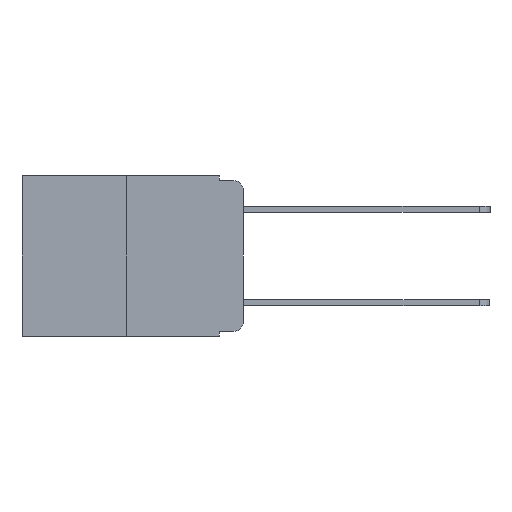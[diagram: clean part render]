
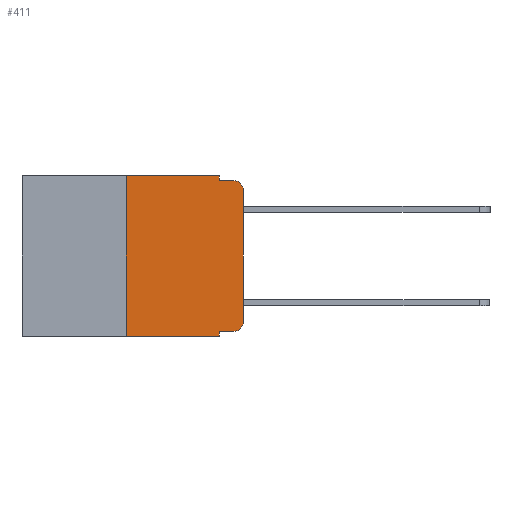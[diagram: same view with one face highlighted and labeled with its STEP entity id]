
A CAD part, left-side view. The second image highlights one B-rep face of the part: STEP entity #411.
In plain terms, the highlighted planar face has unit normal (-1, 0, 0).
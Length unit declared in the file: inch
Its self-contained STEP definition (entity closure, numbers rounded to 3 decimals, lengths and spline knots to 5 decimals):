
#336 = CARTESIAN_POINT ( 'NONE',  ( 0., 0.02, -0.313 ) ) ;
#411 = ADVANCED_FACE ( 'NONE', ( #3045 ), #5713, .F. ) ;
#420 = DIRECTION ( 'NONE',  ( -1., 0., 0. ) ) ;
#532 = DIRECTION ( 'NONE',  ( 0., 0., -1. ) ) ;
#598 = CIRCLE ( 'NONE', #4570, 0.02 ) ;
#1168 = VERTEX_POINT ( 'NONE', #6131 ) ;
#1173 = ORIENTED_EDGE ( 'NONE', *, *, #4968, .T. ) ;
#1184 = LINE ( 'NONE', #3582, #5686 ) ;
#1419 = CARTESIAN_POINT ( 'NONE',  ( 0., 0.051, -0.333 ) ) ;
#1470 = LINE ( 'NONE', #8242, #6229 ) ;
#1533 = VECTOR ( 'NONE', #8042, 39.37008 ) ;
#1577 = ORIENTED_EDGE ( 'NONE', *, *, #6551, .T. ) ;
#2350 = DIRECTION ( 'NONE',  ( 0., 0., -1. ) ) ;
#2496 = CARTESIAN_POINT ( 'NONE',  ( 0., 0.051, -0.343 ) ) ;
#2653 = CARTESIAN_POINT ( 'NONE',  ( 0., 0.25, -0.343 ) ) ;
#2682 = LINE ( 'NONE', #7331, #4887 ) ;
#2841 = CARTESIAN_POINT ( 'NONE',  ( 0., 0.051, -0.01 ) ) ;
#3012 = LINE ( 'NONE', #4731, #4686 ) ;
#3023 = EDGE_CURVE ( 'NONE', #3335, #9179, #1184, .T. ) ;
#3045 = FACE_OUTER_BOUND ( 'NONE', #3827, .T. ) ;
#3048 = VECTOR ( 'NONE', #9003, 39.37008 ) ;
#3119 = DIRECTION ( 'NONE',  ( 0., 0., -1. ) ) ;
#3122 = VERTEX_POINT ( 'NONE', #2841 ) ;
#3273 = VECTOR ( 'NONE', #6348, 39.37008 ) ;
#3335 = VERTEX_POINT ( 'NONE', #1419 ) ;
#3411 = DIRECTION ( 'NONE',  ( 0., 0., 1. ) ) ;
#3552 = ORIENTED_EDGE ( 'NONE', *, *, #3023, .T. ) ;
#3571 = DIRECTION ( 'NONE',  ( 0., -1., 0. ) ) ;
#3582 = CARTESIAN_POINT ( 'NONE',  ( 0., 0.051, -0.333 ) ) ;
#3827 = EDGE_LOOP ( 'NONE', ( #4989, #1577, #6557, #9581, #6448, #9211, #1173, #5614, #3552, #4178 ) ) ;
#3895 = VERTEX_POINT ( 'NONE', #4046 ) ;
#4046 = CARTESIAN_POINT ( 'NONE',  ( 0., 0., -0.313 ) ) ;
#4178 = ORIENTED_EDGE ( 'NONE', *, *, #4675, .T. ) ;
#4570 = AXIS2_PLACEMENT_3D ( 'NONE', #336, #420, #3119 ) ;
#4661 = LINE ( 'NONE', #4848, #1533 ) ;
#4675 = EDGE_CURVE ( 'NONE', #9179, #3895, #598, .T. ) ;
#4686 = VECTOR ( 'NONE', #9486, 39.37008 ) ;
#4731 = CARTESIAN_POINT ( 'NONE',  ( 0., 0.051, 0. ) ) ;
#4745 = CARTESIAN_POINT ( 'NONE',  ( 0., 0.25, 0. ) ) ;
#4848 = CARTESIAN_POINT ( 'NONE',  ( 0., 0.051, -0.01 ) ) ;
#4865 = CARTESIAN_POINT ( 'NONE',  ( 0., 0.473, 0. ) ) ;
#4877 = EDGE_CURVE ( 'NONE', #3895, #1168, #9187, .T. ) ;
#4887 = VECTOR ( 'NONE', #2350, 39.37008 ) ;
#4968 = EDGE_CURVE ( 'NONE', #8646, #6104, #10304, .T. ) ;
#4989 = ORIENTED_EDGE ( 'NONE', *, *, #4877, .T. ) ;
#5466 = LINE ( 'NONE', #7099, #3273 ) ;
#5547 = DIRECTION ( 'NONE',  ( 0., -1., 0. ) ) ;
#5614 = ORIENTED_EDGE ( 'NONE', *, *, #10191, .F. ) ;
#5627 = DIRECTION ( 'NONE',  ( -1., 0., 0. ) ) ;
#5686 = VECTOR ( 'NONE', #3571, 39.37008 ) ;
#5713 = PLANE ( 'NONE',  #9469 ) ;
#6104 = VERTEX_POINT ( 'NONE', #2496 ) ;
#6131 = CARTESIAN_POINT ( 'NONE',  ( 0., 0., -0.03 ) ) ;
#6178 = VECTOR ( 'NONE', #5547, 39.37008 ) ;
#6229 = VECTOR ( 'NONE', #3411, 39.37008 ) ;
#6348 = DIRECTION ( 'NONE',  ( 0., -1., 0. ) ) ;
#6448 = ORIENTED_EDGE ( 'NONE', *, *, #8074, .F. ) ;
#6465 = AXIS2_PLACEMENT_3D ( 'NONE', #10323, #5627, #532 ) ;
#6535 = VERTEX_POINT ( 'NONE', #4745 ) ;
#6551 = EDGE_CURVE ( 'NONE', #1168, #9773, #8550, .T. ) ;
#6557 = ORIENTED_EDGE ( 'NONE', *, *, #7595, .F. ) ;
#6841 = CARTESIAN_POINT ( 'NONE',  ( 0., 0.02, -0.333 ) ) ;
#7099 = CARTESIAN_POINT ( 'NONE',  ( 0., 0.473, 0. ) ) ;
#7331 = CARTESIAN_POINT ( 'NONE',  ( 0., 0.051, 0. ) ) ;
#7595 = EDGE_CURVE ( 'NONE', #3122, #9773, #4661, .T. ) ;
#7635 = CARTESIAN_POINT ( 'NONE',  ( 0., 0.02, -0.01 ) ) ;
#7708 = DIRECTION ( 'NONE',  ( 1., 0., 0. ) ) ;
#8042 = DIRECTION ( 'NONE',  ( 0., -1., 0. ) ) ;
#8074 = EDGE_CURVE ( 'NONE', #6535, #8246, #5466, .T. ) ;
#8105 = EDGE_CURVE ( 'NONE', #8246, #3122, #3012, .T. ) ;
#8126 = CARTESIAN_POINT ( 'NONE',  ( 0., 0.051, 0. ) ) ;
#8242 = CARTESIAN_POINT ( 'NONE',  ( 0., 0.25, 0. ) ) ;
#8246 = VERTEX_POINT ( 'NONE', #8126 ) ;
#8550 = CIRCLE ( 'NONE', #6465, 0.02 ) ;
#8646 = VERTEX_POINT ( 'NONE', #2653 ) ;
#8962 = CARTESIAN_POINT ( 'NONE',  ( 0., 0., 0. ) ) ;
#9003 = DIRECTION ( 'NONE',  ( 0., 0., 1. ) ) ;
#9179 = VERTEX_POINT ( 'NONE', #6841 ) ;
#9187 = LINE ( 'NONE', #8962, #3048 ) ;
#9211 = ORIENTED_EDGE ( 'NONE', *, *, #9661, .F. ) ;
#9248 = DIRECTION ( 'NONE',  ( 0., 0., -1. ) ) ;
#9469 = AXIS2_PLACEMENT_3D ( 'NONE', #4865, #7708, #9248 ) ;
#9486 = DIRECTION ( 'NONE',  ( 0., 0., -1. ) ) ;
#9581 = ORIENTED_EDGE ( 'NONE', *, *, #8105, .F. ) ;
#9661 = EDGE_CURVE ( 'NONE', #8646, #6535, #1470, .T. ) ;
#9677 = CARTESIAN_POINT ( 'NONE',  ( 0., 0.473, -0.343 ) ) ;
#9773 = VERTEX_POINT ( 'NONE', #7635 ) ;
#10191 = EDGE_CURVE ( 'NONE', #3335, #6104, #2682, .T. ) ;
#10304 = LINE ( 'NONE', #9677, #6178 ) ;
#10323 = CARTESIAN_POINT ( 'NONE',  ( 0., 0.02, -0.03 ) ) ;
